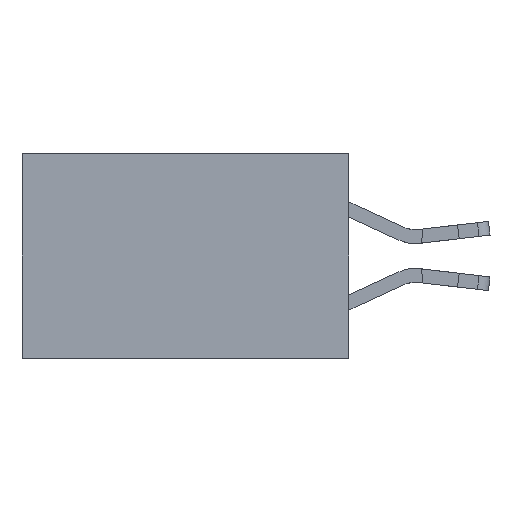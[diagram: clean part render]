
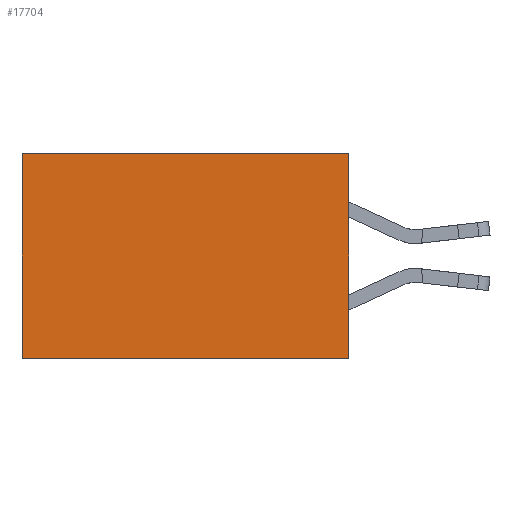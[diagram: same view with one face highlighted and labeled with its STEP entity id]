
A CAD part, left-side view. The second image highlights one B-rep face of the part: STEP entity #17704.
In plain terms, the highlighted planar face has unit normal (-1, 0, 0).
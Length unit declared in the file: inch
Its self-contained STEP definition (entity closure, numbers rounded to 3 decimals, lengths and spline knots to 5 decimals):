
#842 = VERTEX_POINT ( 'NONE', #6170 ) ;
#960 = CARTESIAN_POINT ( 'NONE',  ( 0.277, 0.59, 0. ) ) ;
#1329 = VECTOR ( 'NONE', #4244, 39.37008 ) ;
#1689 = DIRECTION ( 'NONE',  ( 0., 1., 0. ) ) ;
#1796 = ORIENTED_EDGE ( 'NONE', *, *, #6284, .T. ) ;
#2158 = EDGE_CURVE ( 'NONE', #842, #9547, #6328, .T. ) ;
#3520 = EDGE_CURVE ( 'NONE', #6492, #842, #10493, .T. ) ;
#4031 = AXIS2_PLACEMENT_3D ( 'NONE', #16652, #8063, #18013 ) ;
#4244 = DIRECTION ( 'NONE',  ( 0., 1., 0. ) ) ;
#4333 = EDGE_LOOP ( 'NONE', ( #7770, #8781, #9273, #1796 ) ) ;
#5161 = VECTOR ( 'NONE', #6871, 39.37008 ) ;
#5581 = CARTESIAN_POINT ( 'NONE',  ( 0.277, 0., 0. ) ) ;
#6170 = CARTESIAN_POINT ( 'NONE',  ( 0.277, 0., -0.37 ) ) ;
#6284 = EDGE_CURVE ( 'NONE', #6492, #13322, #13096, .T. ) ;
#6328 = LINE ( 'NONE', #9779, #13634 ) ;
#6387 = FACE_OUTER_BOUND ( 'NONE', #4333, .T. ) ;
#6492 = VERTEX_POINT ( 'NONE', #15390 ) ;
#6871 = DIRECTION ( 'NONE',  ( 0., 0., -1. ) ) ;
#7770 = ORIENTED_EDGE ( 'NONE', *, *, #18361, .T. ) ;
#8063 = DIRECTION ( 'NONE',  ( 1., 0., 0. ) ) ;
#8781 = ORIENTED_EDGE ( 'NONE', *, *, #2158, .F. ) ;
#9273 = ORIENTED_EDGE ( 'NONE', *, *, #3520, .F. ) ;
#9547 = VERTEX_POINT ( 'NONE', #13029 ) ;
#9779 = CARTESIAN_POINT ( 'NONE',  ( 0.277, 0., -0.37 ) ) ;
#10493 = LINE ( 'NONE', #13074, #13848 ) ;
#13029 = CARTESIAN_POINT ( 'NONE',  ( 0.277, 0.59, -0.37 ) ) ;
#13074 = CARTESIAN_POINT ( 'NONE',  ( 0.277, 0., -0.37 ) ) ;
#13096 = LINE ( 'NONE', #5581, #1329 ) ;
#13322 = VERTEX_POINT ( 'NONE', #960 ) ;
#13634 = VECTOR ( 'NONE', #1689, 39.37008 ) ;
#13848 = VECTOR ( 'NONE', #14952, 39.37008 ) ;
#14952 = DIRECTION ( 'NONE',  ( 0., 0., -1. ) ) ;
#15170 = PLANE ( 'NONE',  #4031 ) ;
#15390 = CARTESIAN_POINT ( 'NONE',  ( 0.277, 0., 0. ) ) ;
#16652 = CARTESIAN_POINT ( 'NONE',  ( 0.277, 0., -0.37 ) ) ;
#16759 = LINE ( 'NONE', #18288, #5161 ) ;
#17704 = ADVANCED_FACE ( 'NONE', ( #6387 ), #15170, .F. ) ;
#18013 = DIRECTION ( 'NONE',  ( 0., 0., -1. ) ) ;
#18288 = CARTESIAN_POINT ( 'NONE',  ( 0.277, 0.59, -0.37 ) ) ;
#18361 = EDGE_CURVE ( 'NONE', #13322, #9547, #16759, .T. ) ;
